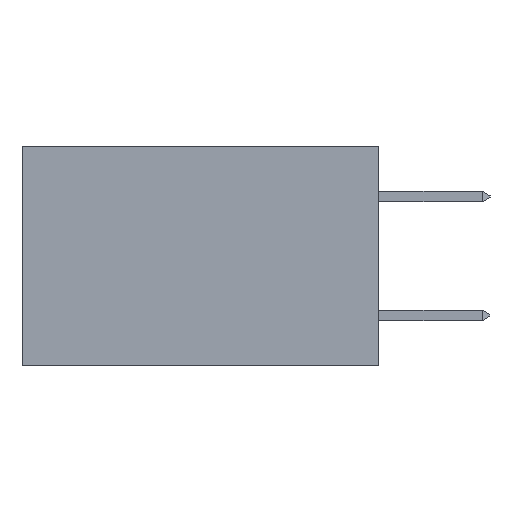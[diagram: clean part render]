
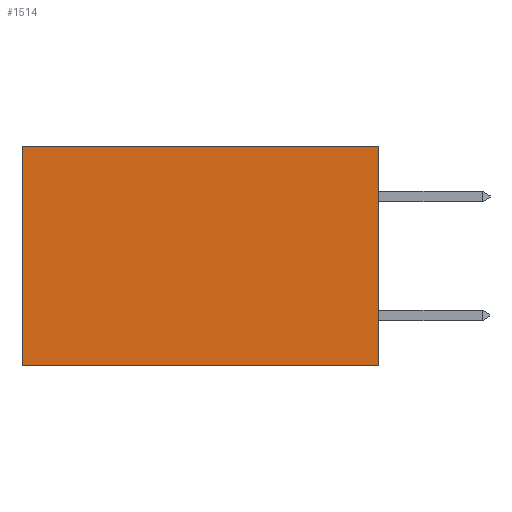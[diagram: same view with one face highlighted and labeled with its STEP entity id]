
A CAD part, left-side view. The second image highlights one B-rep face of the part: STEP entity #1514.
In plain terms, the highlighted planar face has unit normal (-1, 0, 0).
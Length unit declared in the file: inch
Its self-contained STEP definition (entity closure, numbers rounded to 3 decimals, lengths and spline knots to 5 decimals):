
#315 = CARTESIAN_POINT ( 'NONE',  ( 0.298, 0., 0. ) ) ;
#913 = VECTOR ( 'NONE', #4965, 39.37008 ) ;
#1011 = CARTESIAN_POINT ( 'NONE',  ( 0.298, 0., -0.37 ) ) ;
#1169 = LINE ( 'NONE', #1011, #15779 ) ;
#1514 = ADVANCED_FACE ( 'NONE', ( #14313 ), #10775, .F. ) ;
#1643 = LINE ( 'NONE', #11509, #8082 ) ;
#2291 = ORIENTED_EDGE ( 'NONE', *, *, #14893, .T. ) ;
#2313 = ORIENTED_EDGE ( 'NONE', *, *, #8611, .F. ) ;
#2463 = DIRECTION ( 'NONE',  ( 0., 1., 0. ) ) ;
#2606 = ORIENTED_EDGE ( 'NONE', *, *, #3738, .F. ) ;
#3016 = ORIENTED_EDGE ( 'NONE', *, *, #12183, .T. ) ;
#3651 = LINE ( 'NONE', #10061, #12762 ) ;
#3665 = CARTESIAN_POINT ( 'NONE',  ( 0.298, 0.6, 0. ) ) ;
#3738 = EDGE_CURVE ( 'NONE', #5754, #11451, #3651, .T. ) ;
#4965 = DIRECTION ( 'NONE',  ( 0., 0., -1. ) ) ;
#5754 = VERTEX_POINT ( 'NONE', #315 ) ;
#6332 = CARTESIAN_POINT ( 'NONE',  ( 0.298, 0.6, -0.37 ) ) ;
#8082 = VECTOR ( 'NONE', #13881, 39.37008 ) ;
#8280 = VERTEX_POINT ( 'NONE', #14225 ) ;
#8510 = DIRECTION ( 'NONE',  ( 1., 0., 0. ) ) ;
#8611 = EDGE_CURVE ( 'NONE', #11451, #15859, #1169, .T. ) ;
#9251 = DIRECTION ( 'NONE',  ( 0., 0., -1. ) ) ;
#9357 = CARTESIAN_POINT ( 'NONE',  ( 0.298, 0., 0. ) ) ;
#10061 = CARTESIAN_POINT ( 'NONE',  ( 0.298, 0., 0. ) ) ;
#10604 = CARTESIAN_POINT ( 'NONE',  ( 0.298, 0., -0.37 ) ) ;
#10775 = PLANE ( 'NONE',  #11544 ) ;
#11162 = LINE ( 'NONE', #3665, #913 ) ;
#11451 = VERTEX_POINT ( 'NONE', #10604 ) ;
#11509 = CARTESIAN_POINT ( 'NONE',  ( 0.298, 0., 0. ) ) ;
#11544 = AXIS2_PLACEMENT_3D ( 'NONE', #9357, #8510, #9251 ) ;
#12183 = EDGE_CURVE ( 'NONE', #5754, #8280, #1643, .T. ) ;
#12746 = EDGE_LOOP ( 'NONE', ( #2291, #2313, #2606, #3016 ) ) ;
#12762 = VECTOR ( 'NONE', #12908, 39.37008 ) ;
#12908 = DIRECTION ( 'NONE',  ( 0., 0., -1. ) ) ;
#13881 = DIRECTION ( 'NONE',  ( 0., 1., 0. ) ) ;
#14225 = CARTESIAN_POINT ( 'NONE',  ( 0.298, 0.6, 0. ) ) ;
#14313 = FACE_OUTER_BOUND ( 'NONE', #12746, .T. ) ;
#14893 = EDGE_CURVE ( 'NONE', #8280, #15859, #11162, .T. ) ;
#15779 = VECTOR ( 'NONE', #2463, 39.37008 ) ;
#15859 = VERTEX_POINT ( 'NONE', #6332 ) ;
